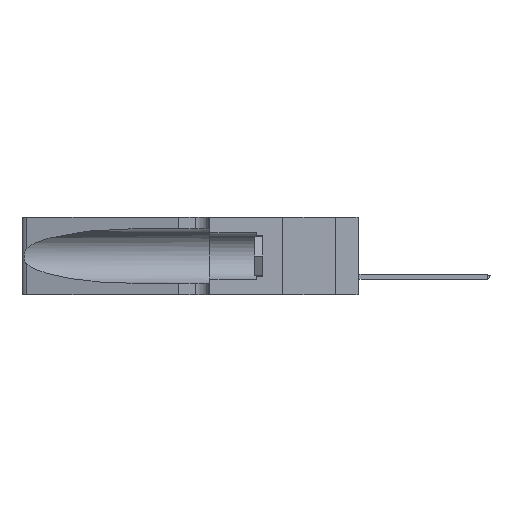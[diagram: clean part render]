
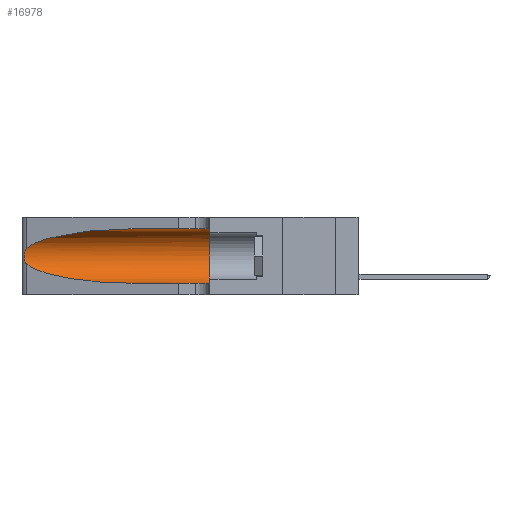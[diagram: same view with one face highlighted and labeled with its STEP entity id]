
A CAD part, left-side view. The second image highlights one B-rep face of the part: STEP entity #16978.
In plain terms, the highlighted cylindrical face has radius 3.308 mm (diameter 6.617 mm), a partial arc.
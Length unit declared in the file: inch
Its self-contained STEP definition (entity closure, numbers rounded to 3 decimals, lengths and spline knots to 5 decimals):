
#29 = FACE_OUTER_BOUND ( 'NONE', #28445, .T. ) ;
#917 = CARTESIAN_POINT ( 'NONE',  ( 0.18966, 0.96281, 0.31525 ) ) ;
#1195 = CARTESIAN_POINT ( 'NONE',  ( 0.25854, 1.2359, 0.20912 ) ) ;
#1654 = DIRECTION ( 'NONE',  ( 0., -1., 0. ) ) ;
#1788 = VECTOR ( 'NONE', #1654, 39.37008 ) ;
#1789 = VERTEX_POINT ( 'NONE', #18871 ) ;
#2990 = CARTESIAN_POINT ( 'NONE',  ( 0.1305, 1.61858, 0.185 ) ) ;
#3392 = AXIS2_PLACEMENT_3D ( 'NONE', #2990, #20745, #22538 ) ;
#3574 = ORIENTED_EDGE ( 'NONE', *, *, #29583, .F. ) ;
#4182 = CARTESIAN_POINT ( 'NONE',  ( 0.26075, 1.23896, 0.178 ) ) ;
#4286 = CARTESIAN_POINT ( 'NONE',  ( 0.25639, 1.23184, 0.21858 ) ) ;
#4389 = CARTESIAN_POINT ( 'NONE',  ( 0.25787, 1.23484, 0.2124 ) ) ;
#4970 = CARTESIAN_POINT ( 'NONE',  ( 0.1305, 0.72297, 0.05475 ) ) ;
#5060 = AXIS2_PLACEMENT_3D ( 'NONE', #29015, #16778, #21835 ) ;
#5794 =( BOUNDED_CURVE ( )  B_SPLINE_CURVE ( 3, ( #27092, #17354, #19832, #4970 ),
 .UNSPECIFIED., .F., .T. ) 
 B_SPLINE_CURVE_WITH_KNOTS ( ( 4, 4 ),
 ( 3.44316, 4.71239 ),
 .UNSPECIFIED. ) 
 CURVE ( )  GEOMETRIC_REPRESENTATION_ITEM ( )  RATIONAL_B_SPLINE_CURVE ( ( 1., 0.87, 0.87, 1. ) ) 
 REPRESENTATION_ITEM ( '' )  );
#6007 = CARTESIAN_POINT ( 'NONE',  ( 0.26017, 1.23833, 0.17102 ) ) ;
#6493 = LINE ( 'NONE', #29134, #1788 ) ;
#6702 = CARTESIAN_POINT ( 'NONE',  ( 0.25487, 1.22718, 0.14631 ) ) ;
#7071 = LINE ( 'NONE', #12454, #20591 ) ;
#7374 = VERTEX_POINT ( 'NONE', #11574 ) ;
#8330 = CIRCLE ( 'NONE', #5060, 0.13025 ) ;
#8490 = CARTESIAN_POINT ( 'NONE',  ( 0.25639, 1.23186, 0.15144 ) ) ;
#8866 = ORIENTED_EDGE ( 'NONE', *, *, #21752, .T. ) ;
#9170 = CARTESIAN_POINT ( 'NONE',  ( 0.25555, 1.22993, 0.14849 ) ) ;
#9383 = CARTESIAN_POINT ( 'NONE',  ( 0.25555, 1.22994, 0.2215 ) ) ;
#9473 = EDGE_CURVE ( 'NONE', #24952, #1789, #30097, .T. ) ;
#11510 = VERTEX_POINT ( 'NONE', #29186 ) ;
#11574 = CARTESIAN_POINT ( 'NONE',  ( 0.1305, 0.72297, 0.31525 ) ) ;
#11770 = CARTESIAN_POINT ( 'NONE',  ( 0.26075, 1.23896, 0.19203 ) ) ;
#12454 = CARTESIAN_POINT ( 'NONE',  ( 0.1305, 1.61858, 0.05475 ) ) ;
#13688 = CARTESIAN_POINT ( 'NONE',  ( 0.1305, 0.72297, 0.05475 ) ) ;
#15253 = CARTESIAN_POINT ( 'NONE',  ( 0.25487, 1.22718, 0.22369 ) ) ;
#16778 = DIRECTION ( 'NONE',  ( 0., 1., 0. ) ) ;
#16978 = ADVANCED_FACE ( 'NONE', ( #29 ), #21010, .F. ) ;
#17354 = CARTESIAN_POINT ( 'NONE',  ( 0.2373, 1.15595, 0.08982 ) ) ;
#18871 = CARTESIAN_POINT ( 'NONE',  ( 0.25487, 1.22718, 0.14631 ) ) ;
#19832 = CARTESIAN_POINT ( 'NONE',  ( 0.18966, 0.96281, 0.05475 ) ) ;
#20508 = VERTEX_POINT ( 'NONE', #13688 ) ;
#20591 = VECTOR ( 'NONE', #22812, 39.37008 ) ;
#20745 = DIRECTION ( 'NONE',  ( 0., -1., 0. ) ) ;
#21010 = CYLINDRICAL_SURFACE ( 'NONE', #3392, 0.13025 ) ;
#21518 = CARTESIAN_POINT ( 'NONE',  ( 0.25487, 1.22718, 0.22369 ) ) ;
#21636 = CARTESIAN_POINT ( 'NONE',  ( 0.26018, 1.23835, 0.19895 ) ) ;
#21729 = CARTESIAN_POINT ( 'NONE',  ( 0.25789, 1.23486, 0.15765 ) ) ;
#21752 = EDGE_CURVE ( 'NONE', #7374, #24952, #24325, .T. ) ;
#21777 = ORIENTED_EDGE ( 'NONE', *, *, #9473, .T. ) ;
#21835 = DIRECTION ( 'NONE',  ( 0., 0., 1. ) ) ;
#21869 = ORIENTED_EDGE ( 'NONE', *, *, #26292, .T. ) ;
#22538 = DIRECTION ( 'NONE',  ( 0., 0., -1. ) ) ;
#22550 = ORIENTED_EDGE ( 'NONE', *, *, #26315, .T. ) ;
#22741 = EDGE_CURVE ( 'NONE', #7374, #27233, #6493, .T. ) ;
#22812 = DIRECTION ( 'NONE',  ( 0., -1., 0. ) ) ;
#23376 = CARTESIAN_POINT ( 'NONE',  ( 0.2373, 1.15595, 0.28018 ) ) ;
#24325 =( BOUNDED_CURVE ( )  B_SPLINE_CURVE ( 3, ( #25164, #917, #23376, #25727 ),
 .UNSPECIFIED., .F., .F. ) 
 B_SPLINE_CURVE_WITH_KNOTS ( ( 4, 4 ),
 ( 1.5708, 2.84003 ),
 .UNSPECIFIED. ) 
 CURVE ( )  GEOMETRIC_REPRESENTATION_ITEM ( )  RATIONAL_B_SPLINE_CURVE ( ( 1., 0.87, 0.87, 1. ) ) 
 REPRESENTATION_ITEM ( '' )  );
#24952 = VERTEX_POINT ( 'NONE', #15253 ) ;
#25164 = CARTESIAN_POINT ( 'NONE',  ( 0.1305, 0.72297, 0.31525 ) ) ;
#25579 = CARTESIAN_POINT ( 'NONE',  ( 0.1305, 0.35, 0.31525 ) ) ;
#25727 = CARTESIAN_POINT ( 'NONE',  ( 0.25487, 1.22718, 0.22369 ) ) ;
#26292 = EDGE_CURVE ( 'NONE', #1789, #20508, #5794, .T. ) ;
#26315 = EDGE_CURVE ( 'NONE', #20508, #11510, #7071, .T. ) ;
#27092 = CARTESIAN_POINT ( 'NONE',  ( 0.25487, 1.22718, 0.14631 ) ) ;
#27233 = VERTEX_POINT ( 'NONE', #25579 ) ;
#28445 = EDGE_LOOP ( 'NONE', ( #8866, #21777, #21869, #22550, #3574, #28611 ) ) ;
#28611 = ORIENTED_EDGE ( 'NONE', *, *, #22741, .F. ) ;
#29015 = CARTESIAN_POINT ( 'NONE',  ( 0.1305, 0.35, 0.185 ) ) ;
#29134 = CARTESIAN_POINT ( 'NONE',  ( 0.1305, 1.61858, 0.31525 ) ) ;
#29186 = CARTESIAN_POINT ( 'NONE',  ( 0.1305, 0.35, 0.05475 ) ) ;
#29583 = EDGE_CURVE ( 'NONE', #27233, #11510, #8330, .T. ) ;
#30097 = B_SPLINE_CURVE_WITH_KNOTS ( 'NONE', 3,
 ( #21518, #9383, #4286, #4389, #1195, #21636, #11770, #4182, #6007, #31492, #21729, #8490, #9170, #6702 ),
 .UNSPECIFIED., .F., .F.,
 ( 4, 2, 2, 2, 2, 2, 4 ),
 ( 0., 0.00027, 0.00053, 0.00107, 0.0016, 0.00187, 0.00214 ),
 .UNSPECIFIED. ) ;
#31492 = CARTESIAN_POINT ( 'NONE',  ( 0.25856, 1.23593, 0.16098 ) ) ;
